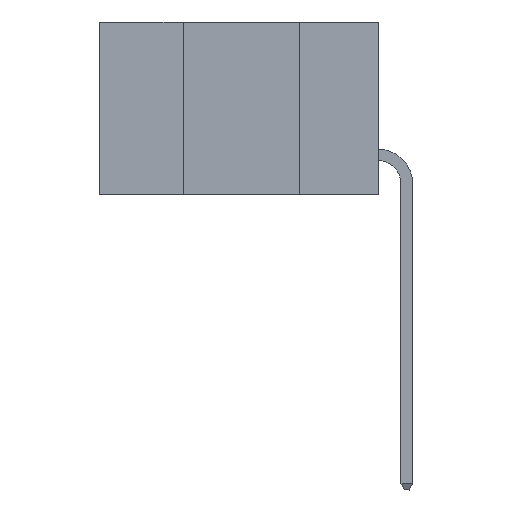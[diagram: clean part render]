
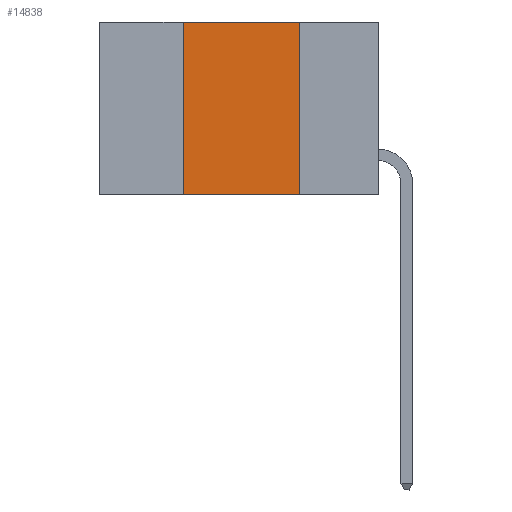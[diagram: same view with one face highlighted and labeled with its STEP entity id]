
A CAD part, left-side view. The second image highlights one B-rep face of the part: STEP entity #14838.
In plain terms, the highlighted planar face has unit normal (-1, 0, 0).
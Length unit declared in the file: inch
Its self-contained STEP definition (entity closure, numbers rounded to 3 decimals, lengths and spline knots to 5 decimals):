
#335 = CARTESIAN_POINT ( 'NONE',  ( 0., 0.42, -0.37 ) ) ;
#568 = ORIENTED_EDGE ( 'NONE', *, *, #11408, .F. ) ;
#880 = VERTEX_POINT ( 'NONE', #7536 ) ;
#1655 = VECTOR ( 'NONE', #18303, 39.37008 ) ;
#2934 = CARTESIAN_POINT ( 'NONE',  ( 0., 0.6, 0. ) ) ;
#4204 = VERTEX_POINT ( 'NONE', #15922 ) ;
#5219 = LINE ( 'NONE', #20574, #15910 ) ;
#6104 = ORIENTED_EDGE ( 'NONE', *, *, #16008, .F. ) ;
#6553 = CARTESIAN_POINT ( 'NONE',  ( 0., 0.17, -0.37 ) ) ;
#7536 = CARTESIAN_POINT ( 'NONE',  ( 0., 0.42, 0. ) ) ;
#8828 = EDGE_CURVE ( 'NONE', #4204, #880, #21683, .T. ) ;
#9570 = ORIENTED_EDGE ( 'NONE', *, *, #8828, .F. ) ;
#9969 = PLANE ( 'NONE',  #17693 ) ;
#10400 = DIRECTION ( 'NONE',  ( 0., 0., -1. ) ) ;
#10648 = EDGE_CURVE ( 'NONE', #4204, #11061, #5219, .T. ) ;
#11061 = VERTEX_POINT ( 'NONE', #20307 ) ;
#11408 = EDGE_CURVE ( 'NONE', #880, #11894, #19905, .T. ) ;
#11588 = CARTESIAN_POINT ( 'NONE',  ( 0., 0.6, 0. ) ) ;
#11894 = VERTEX_POINT ( 'NONE', #18362 ) ;
#12278 = LINE ( 'NONE', #6553, #12595 ) ;
#12595 = VECTOR ( 'NONE', #10400, 39.37008 ) ;
#12671 = DIRECTION ( 'NONE',  ( 0., -1., 0. ) ) ;
#13690 = DIRECTION ( 'NONE',  ( 0., 0., -1. ) ) ;
#14779 = DIRECTION ( 'NONE',  ( 0., 0., 1. ) ) ;
#14838 = ADVANCED_FACE ( 'NONE', ( #19372 ), #9969, .F. ) ;
#15207 = ORIENTED_EDGE ( 'NONE', *, *, #10648, .T. ) ;
#15297 = DIRECTION ( 'NONE',  ( 1., 0., 0. ) ) ;
#15910 = VECTOR ( 'NONE', #12671, 39.37008 ) ;
#15922 = CARTESIAN_POINT ( 'NONE',  ( 0., 0.42, -0.37 ) ) ;
#16008 = EDGE_CURVE ( 'NONE', #11894, #11061, #12278, .T. ) ;
#17693 = AXIS2_PLACEMENT_3D ( 'NONE', #11588, #15297, #13690 ) ;
#18303 = DIRECTION ( 'NONE',  ( 0., -1., 0. ) ) ;
#18362 = CARTESIAN_POINT ( 'NONE',  ( 0., 0.17, 0. ) ) ;
#18647 = EDGE_LOOP ( 'NONE', ( #6104, #568, #9570, #15207 ) ) ;
#19372 = FACE_OUTER_BOUND ( 'NONE', #18647, .T. ) ;
#19905 = LINE ( 'NONE', #2934, #1655 ) ;
#20307 = CARTESIAN_POINT ( 'NONE',  ( 0., 0.17, -0.37 ) ) ;
#20574 = CARTESIAN_POINT ( 'NONE',  ( 0., 0.6, -0.37 ) ) ;
#20939 = VECTOR ( 'NONE', #14779, 39.37008 ) ;
#21683 = LINE ( 'NONE', #335, #20939 ) ;
